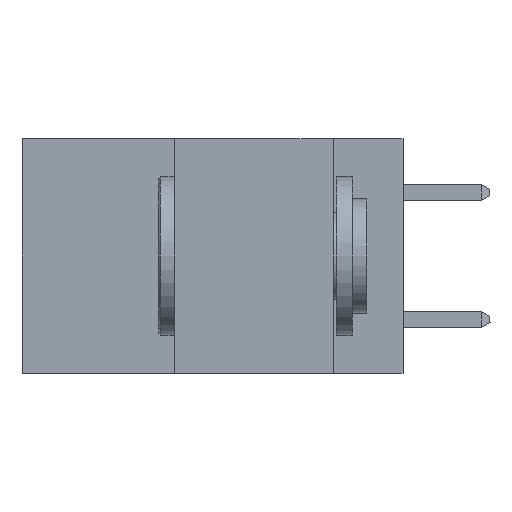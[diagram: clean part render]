
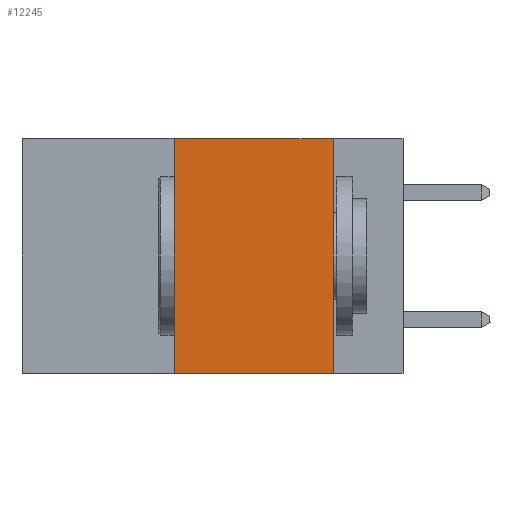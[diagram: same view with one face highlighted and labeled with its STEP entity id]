
A CAD part, left-side view. The second image highlights one B-rep face of the part: STEP entity #12245.
In plain terms, the highlighted planar face has unit normal (-1, 0, 0).
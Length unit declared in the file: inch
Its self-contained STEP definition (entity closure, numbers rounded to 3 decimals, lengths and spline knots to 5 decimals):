
#515 = LINE ( 'NONE', #13096, #37216 ) ;
#766 = CARTESIAN_POINT ( 'NONE',  ( 0., 0.36, 0. ) ) ;
#4659 = CARTESIAN_POINT ( 'NONE',  ( 0., 0.11, 0. ) ) ;
#4808 = CARTESIAN_POINT ( 'NONE',  ( 0., 0.6, 0. ) ) ;
#6122 = VECTOR ( 'NONE', #6191, 39.37008 ) ;
#6191 = DIRECTION ( 'NONE',  ( 0., -1., 0. ) ) ;
#7339 = VERTEX_POINT ( 'NONE', #23518 ) ;
#7976 = DIRECTION ( 'NONE',  ( 0., -1., 0. ) ) ;
#8363 = CARTESIAN_POINT ( 'NONE',  ( 0., 0.36, -0.37 ) ) ;
#8826 = DIRECTION ( 'NONE',  ( 1., 0., 0. ) ) ;
#9088 = LINE ( 'NONE', #43614, #19867 ) ;
#11510 = EDGE_CURVE ( 'NONE', #29210, #7339, #9088, .T. ) ;
#12195 = VERTEX_POINT ( 'NONE', #8363 ) ;
#12245 = ADVANCED_FACE ( 'NONE', ( #38433 ), #33801, .F. ) ;
#12506 = DIRECTION ( 'NONE',  ( 0., 0., -1. ) ) ;
#13096 = CARTESIAN_POINT ( 'NONE',  ( 0., 0.36, 0. ) ) ;
#13367 = EDGE_CURVE ( 'NONE', #30572, #29210, #39670, .T. ) ;
#14592 = AXIS2_PLACEMENT_3D ( 'NONE', #15967, #8826, #12506 ) ;
#14693 = EDGE_LOOP ( 'NONE', ( #43348, #15328, #37362, #37622 ) ) ;
#15328 = ORIENTED_EDGE ( 'NONE', *, *, #13367, .F. ) ;
#15967 = CARTESIAN_POINT ( 'NONE',  ( 0., 0.6, 0. ) ) ;
#16896 = DIRECTION ( 'NONE',  ( 0., 0., 1. ) ) ;
#19867 = VECTOR ( 'NONE', #28609, 39.37008 ) ;
#20437 = CARTESIAN_POINT ( 'NONE',  ( 0., 0.6, -0.37 ) ) ;
#23518 = CARTESIAN_POINT ( 'NONE',  ( 0., 0.11, -0.37 ) ) ;
#28265 = EDGE_CURVE ( 'NONE', #12195, #7339, #35004, .T. ) ;
#28609 = DIRECTION ( 'NONE',  ( 0., 0., -1. ) ) ;
#29210 = VERTEX_POINT ( 'NONE', #4659 ) ;
#30572 = VERTEX_POINT ( 'NONE', #766 ) ;
#31187 = VECTOR ( 'NONE', #7976, 39.37008 ) ;
#33801 = PLANE ( 'NONE',  #14592 ) ;
#35004 = LINE ( 'NONE', #20437, #6122 ) ;
#37216 = VECTOR ( 'NONE', #16896, 39.37008 ) ;
#37362 = ORIENTED_EDGE ( 'NONE', *, *, #39682, .F. ) ;
#37622 = ORIENTED_EDGE ( 'NONE', *, *, #28265, .T. ) ;
#38433 = FACE_OUTER_BOUND ( 'NONE', #14693, .T. ) ;
#39670 = LINE ( 'NONE', #4808, #31187 ) ;
#39682 = EDGE_CURVE ( 'NONE', #12195, #30572, #515, .T. ) ;
#43348 = ORIENTED_EDGE ( 'NONE', *, *, #11510, .F. ) ;
#43614 = CARTESIAN_POINT ( 'NONE',  ( 0., 0.11, 0. ) ) ;
